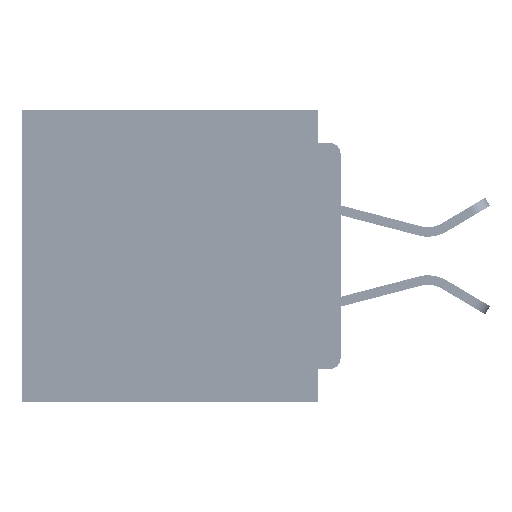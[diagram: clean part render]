
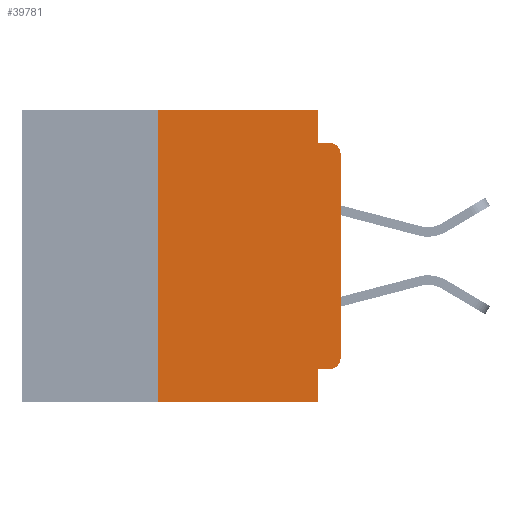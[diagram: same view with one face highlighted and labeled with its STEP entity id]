
A CAD part, left-side view. The second image highlights one B-rep face of the part: STEP entity #39781.
In plain terms, the highlighted planar face has unit normal (-1, 0, 0).
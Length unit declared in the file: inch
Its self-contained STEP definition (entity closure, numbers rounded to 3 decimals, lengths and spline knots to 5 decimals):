
#431 = EDGE_CURVE ( 'NONE', #15178, #3264, #23908, .T. ) ;
#942 = EDGE_CURVE ( 'NONE', #3313, #35860, #58585, .T. ) ;
#1143 = VERTEX_POINT ( 'NONE', #11693 ) ;
#1657 = FACE_OUTER_BOUND ( 'NONE', #35240, .T. ) ;
#2267 = DIRECTION ( 'NONE',  ( 1., 0., 0. ) ) ;
#3264 = VERTEX_POINT ( 'NONE', #47213 ) ;
#3313 = VERTEX_POINT ( 'NONE', #56661 ) ;
#3835 = DIRECTION ( 'NONE',  ( 0., 0., 1. ) ) ;
#4902 = VECTOR ( 'NONE', #8935, 39.37008 ) ;
#4917 = EDGE_CURVE ( 'NONE', #51993, #19131, #58903, .T. ) ;
#5533 = DIRECTION ( 'NONE',  ( 0., 0., 1. ) ) ;
#6848 = CARTESIAN_POINT ( 'NONE',  ( 0., 0.015, -0.06 ) ) ;
#7348 = DIRECTION ( 'NONE',  ( 0., -1., 0. ) ) ;
#7381 = EDGE_CURVE ( 'NONE', #3264, #10223, #17086, .T. ) ;
#7916 = ORIENTED_EDGE ( 'NONE', *, *, #37536, .T. ) ;
#8935 = DIRECTION ( 'NONE',  ( 0., -1., 0. ) ) ;
#9958 = ORIENTED_EDGE ( 'NONE', *, *, #21001, .T. ) ;
#10223 = VERTEX_POINT ( 'NONE', #37080 ) ;
#10284 = VECTOR ( 'NONE', #5533, 39.37008 ) ;
#11473 = DIRECTION ( 'NONE',  ( 0., 0., -1. ) ) ;
#11693 = CARTESIAN_POINT ( 'NONE',  ( 0., 0., -0.34 ) ) ;
#13730 = EDGE_CURVE ( 'NONE', #15381, #10223, #46950, .T. ) ;
#15178 = VERTEX_POINT ( 'NONE', #21560 ) ;
#15374 = LINE ( 'NONE', #44938, #26033 ) ;
#15381 = VERTEX_POINT ( 'NONE', #18192 ) ;
#15883 = PLANE ( 'NONE',  #47503 ) ;
#17086 = LINE ( 'NONE', #58762, #4902 ) ;
#18192 = CARTESIAN_POINT ( 'NONE',  ( 0., 0., -0.06 ) ) ;
#19131 = VERTEX_POINT ( 'NONE', #53795 ) ;
#19383 = AXIS2_PLACEMENT_3D ( 'NONE', #51681, #24535, #56219 ) ;
#19537 = CARTESIAN_POINT ( 'NONE',  ( 0., 0.015, -0.355 ) ) ;
#20037 = VECTOR ( 'NONE', #7348, 39.37008 ) ;
#20364 = CARTESIAN_POINT ( 'NONE',  ( 0., 0.031, 0. ) ) ;
#20393 = CIRCLE ( 'NONE', #19383, 0.015 ) ;
#21001 = EDGE_CURVE ( 'NONE', #3313, #26396, #21458, .T. ) ;
#21458 = LINE ( 'NONE', #34606, #20037 ) ;
#21560 = CARTESIAN_POINT ( 'NONE',  ( 0., 0.031, 0. ) ) ;
#22034 = CARTESIAN_POINT ( 'NONE',  ( 0., 0., 0. ) ) ;
#22280 = ORIENTED_EDGE ( 'NONE', *, *, #13730, .T. ) ;
#23525 = CARTESIAN_POINT ( 'NONE',  ( 0., 0.25, -0.4 ) ) ;
#23908 = LINE ( 'NONE', #20364, #28184 ) ;
#24535 = DIRECTION ( 'NONE',  ( -1., 0., 0. ) ) ;
#25699 = AXIS2_PLACEMENT_3D ( 'NONE', #6848, #38671, #11473 ) ;
#26033 = VECTOR ( 'NONE', #58584, 39.37008 ) ;
#26191 = ORIENTED_EDGE ( 'NONE', *, *, #39354, .F. ) ;
#26396 = VERTEX_POINT ( 'NONE', #57679 ) ;
#27459 = LINE ( 'NONE', #42935, #38056 ) ;
#28184 = VECTOR ( 'NONE', #38397, 39.37008 ) ;
#29619 = CARTESIAN_POINT ( 'NONE',  ( 0., 0.437, 0. ) ) ;
#32564 = CARTESIAN_POINT ( 'NONE',  ( 0., 0., -0.355 ) ) ;
#34132 = ORIENTED_EDGE ( 'NONE', *, *, #54745, .F. ) ;
#34147 = DIRECTION ( 'NONE',  ( 0., 0., -1. ) ) ;
#34606 = CARTESIAN_POINT ( 'NONE',  ( 0., 0.437, -0.4 ) ) ;
#34766 = VECTOR ( 'NONE', #3835, 39.37008 ) ;
#35240 = EDGE_LOOP ( 'NONE', ( #7916, #22280, #55635, #36225, #26191, #43625, #9958, #34132, #55504, #52286 ) ) ;
#35860 = VERTEX_POINT ( 'NONE', #50563 ) ;
#36225 = ORIENTED_EDGE ( 'NONE', *, *, #431, .F. ) ;
#37080 = CARTESIAN_POINT ( 'NONE',  ( 0., 0.015, -0.045 ) ) ;
#37536 = EDGE_CURVE ( 'NONE', #1143, #15381, #46863, .T. ) ;
#38056 = VECTOR ( 'NONE', #52224, 39.37008 ) ;
#38397 = DIRECTION ( 'NONE',  ( 0., 0., -1. ) ) ;
#38671 = DIRECTION ( 'NONE',  ( -1., 0., 0. ) ) ;
#39045 = EDGE_CURVE ( 'NONE', #51993, #1143, #20393, .T. ) ;
#39354 = EDGE_CURVE ( 'NONE', #35860, #15178, #15374, .T. ) ;
#39781 = ADVANCED_FACE ( 'NONE', ( #1657 ), #15883, .F. ) ;
#41699 = DIRECTION ( 'NONE',  ( 0., 1., 0. ) ) ;
#42935 = CARTESIAN_POINT ( 'NONE',  ( 0., 0.031, -0.4 ) ) ;
#43625 = ORIENTED_EDGE ( 'NONE', *, *, #942, .F. ) ;
#44938 = CARTESIAN_POINT ( 'NONE',  ( 0., 0.437, 0. ) ) ;
#46849 = VECTOR ( 'NONE', #41699, 39.37008 ) ;
#46863 = LINE ( 'NONE', #22034, #34766 ) ;
#46950 = CIRCLE ( 'NONE', #25699, 0.015 ) ;
#47213 = CARTESIAN_POINT ( 'NONE',  ( 0., 0.031, -0.045 ) ) ;
#47503 = AXIS2_PLACEMENT_3D ( 'NONE', #29619, #2267, #34147 ) ;
#50563 = CARTESIAN_POINT ( 'NONE',  ( 0., 0.25, 0. ) ) ;
#51681 = CARTESIAN_POINT ( 'NONE',  ( 0., 0.015, -0.34 ) ) ;
#51993 = VERTEX_POINT ( 'NONE', #19537 ) ;
#52224 = DIRECTION ( 'NONE',  ( 0., 0., -1. ) ) ;
#52286 = ORIENTED_EDGE ( 'NONE', *, *, #39045, .T. ) ;
#53795 = CARTESIAN_POINT ( 'NONE',  ( 0., 0.031, -0.355 ) ) ;
#54745 = EDGE_CURVE ( 'NONE', #19131, #26396, #27459, .T. ) ;
#55504 = ORIENTED_EDGE ( 'NONE', *, *, #4917, .F. ) ;
#55635 = ORIENTED_EDGE ( 'NONE', *, *, #7381, .F. ) ;
#56219 = DIRECTION ( 'NONE',  ( 0., 0., -1. ) ) ;
#56661 = CARTESIAN_POINT ( 'NONE',  ( 0., 0.25, -0.4 ) ) ;
#57679 = CARTESIAN_POINT ( 'NONE',  ( 0., 0.031, -0.4 ) ) ;
#58584 = DIRECTION ( 'NONE',  ( 0., -1., 0. ) ) ;
#58585 = LINE ( 'NONE', #23525, #10284 ) ;
#58762 = CARTESIAN_POINT ( 'NONE',  ( 0., 0., -0.045 ) ) ;
#58903 = LINE ( 'NONE', #32564, #46849 ) ;
